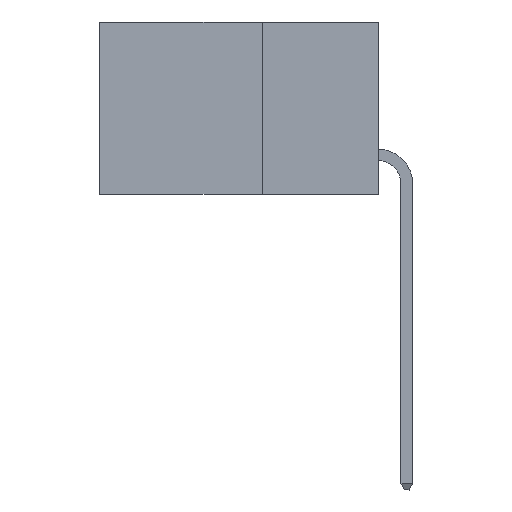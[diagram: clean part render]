
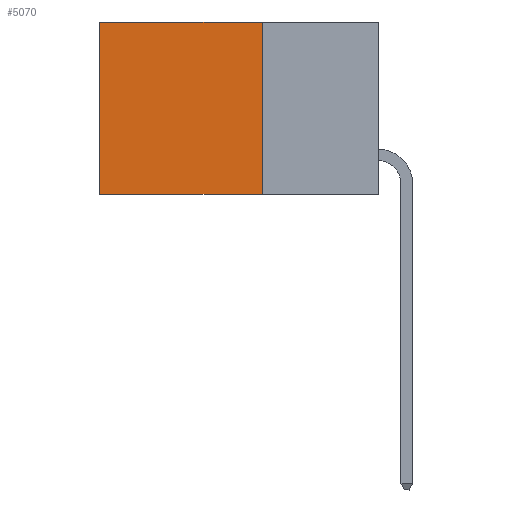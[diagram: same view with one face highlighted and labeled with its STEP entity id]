
A CAD part, left-side view. The second image highlights one B-rep face of the part: STEP entity #5070.
In plain terms, the highlighted planar face has unit normal (-1, 0, 0).
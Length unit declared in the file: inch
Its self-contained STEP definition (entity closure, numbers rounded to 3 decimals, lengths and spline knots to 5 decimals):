
#199 = EDGE_CURVE ( 'NONE', #3778, #7543, #10134, .T. ) ;
#287 = PLANE ( 'NONE',  #4392 ) ;
#592 = EDGE_LOOP ( 'NONE', ( #7811, #5572, #5580, #6174 ) ) ;
#864 = VECTOR ( 'NONE', #3396, 39.37008 ) ;
#891 = LINE ( 'NONE', #8527, #9300 ) ;
#939 = DIRECTION ( 'NONE',  ( 0., 0., -1. ) ) ;
#1134 = CARTESIAN_POINT ( 'NONE',  ( 0.2615, 0.25, -0.37 ) ) ;
#2325 = VERTEX_POINT ( 'NONE', #3991 ) ;
#2678 = CARTESIAN_POINT ( 'NONE',  ( 0.2615, 0.6, 0. ) ) ;
#2828 = DIRECTION ( 'NONE',  ( 1., 0., 0. ) ) ;
#3000 = VECTOR ( 'NONE', #7051, 39.37008 ) ;
#3004 = EDGE_CURVE ( 'NONE', #2325, #7543, #7724, .T. ) ;
#3315 = EDGE_CURVE ( 'NONE', #5112, #3778, #9272, .T. ) ;
#3396 = DIRECTION ( 'NONE',  ( 0., 0., -1. ) ) ;
#3778 = VERTEX_POINT ( 'NONE', #2678 ) ;
#3991 = CARTESIAN_POINT ( 'NONE',  ( 0.2615, 0.25, -0.37 ) ) ;
#4392 = AXIS2_PLACEMENT_3D ( 'NONE', #9663, #2828, #6217 ) ;
#4421 = EDGE_CURVE ( 'NONE', #5112, #2325, #891, .T. ) ;
#5070 = ADVANCED_FACE ( 'NONE', ( #6110 ), #287, .F. ) ;
#5112 = VERTEX_POINT ( 'NONE', #9962 ) ;
#5572 = ORIENTED_EDGE ( 'NONE', *, *, #3004, .F. ) ;
#5580 = ORIENTED_EDGE ( 'NONE', *, *, #4421, .F. ) ;
#5886 = CARTESIAN_POINT ( 'NONE',  ( 0.2615, 0.6, -0.37 ) ) ;
#6110 = FACE_OUTER_BOUND ( 'NONE', #592, .T. ) ;
#6174 = ORIENTED_EDGE ( 'NONE', *, *, #3315, .T. ) ;
#6217 = DIRECTION ( 'NONE',  ( 0., 0., -1. ) ) ;
#6560 = VECTOR ( 'NONE', #8441, 39.37008 ) ;
#7051 = DIRECTION ( 'NONE',  ( 0., 1., 0. ) ) ;
#7543 = VERTEX_POINT ( 'NONE', #10077 ) ;
#7724 = LINE ( 'NONE', #1134, #3000 ) ;
#7811 = ORIENTED_EDGE ( 'NONE', *, *, #199, .T. ) ;
#8285 = CARTESIAN_POINT ( 'NONE',  ( 0.2615, 0.25, 0. ) ) ;
#8441 = DIRECTION ( 'NONE',  ( 0., 1., 0. ) ) ;
#8527 = CARTESIAN_POINT ( 'NONE',  ( 0.2615, 0.25, -0.37 ) ) ;
#9272 = LINE ( 'NONE', #8285, #6560 ) ;
#9300 = VECTOR ( 'NONE', #939, 39.37008 ) ;
#9663 = CARTESIAN_POINT ( 'NONE',  ( 0.2615, 0.25, -0.37 ) ) ;
#9962 = CARTESIAN_POINT ( 'NONE',  ( 0.2615, 0.25, 0. ) ) ;
#10077 = CARTESIAN_POINT ( 'NONE',  ( 0.2615, 0.6, -0.37 ) ) ;
#10134 = LINE ( 'NONE', #5886, #864 ) ;
